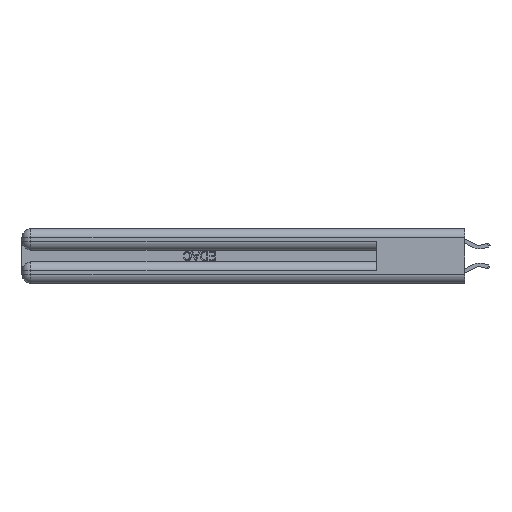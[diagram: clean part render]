
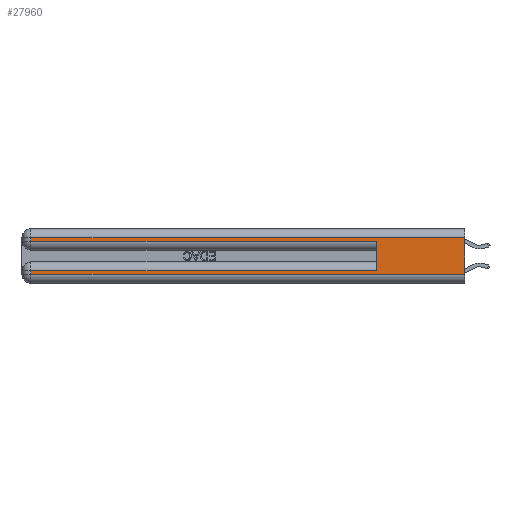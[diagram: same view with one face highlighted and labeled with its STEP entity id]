
A CAD part, left-side view. The second image highlights one B-rep face of the part: STEP entity #27960.
In plain terms, the highlighted planar face has unit normal (-1, 0, 0).
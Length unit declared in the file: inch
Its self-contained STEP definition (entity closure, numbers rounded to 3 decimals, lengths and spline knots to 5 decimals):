
#130 = LINE ( 'NONE', #24938, #30496 ) ;
#816 = LINE ( 'NONE', #9879, #31984 ) ;
#1373 = VECTOR ( 'NONE', #23966, 39.37008 ) ;
#2949 = DIRECTION ( 'NONE',  ( 0., 0., 1. ) ) ;
#3245 = EDGE_CURVE ( 'NONE', #4053, #3680, #5400, .T. ) ;
#3680 = VERTEX_POINT ( 'NONE', #26156 ) ;
#3933 = EDGE_CURVE ( 'NONE', #4053, #18647, #4117, .T. ) ;
#4053 = VERTEX_POINT ( 'NONE', #16327 ) ;
#4099 = CARTESIAN_POINT ( 'NONE',  ( 0., 2.94, 0.31 ) ) ;
#4117 = LINE ( 'NONE', #5490, #31559 ) ;
#4301 = CARTESIAN_POINT ( 'NONE',  ( 0., 0., 0.06 ) ) ;
#5032 = ORIENTED_EDGE ( 'NONE', *, *, #28928, .T. ) ;
#5400 = LINE ( 'NONE', #34355, #10817 ) ;
#5490 = CARTESIAN_POINT ( 'NONE',  ( 0., 0.6, 0.145 ) ) ;
#5714 = VERTEX_POINT ( 'NONE', #21683 ) ;
#5904 = VERTEX_POINT ( 'NONE', #4301 ) ;
#6257 = DIRECTION ( 'NONE',  ( 0., 0., -1. ) ) ;
#7238 = LINE ( 'NONE', #32750, #31319 ) ;
#7413 = DIRECTION ( 'NONE',  ( 0., -1., 0. ) ) ;
#7583 = CARTESIAN_POINT ( 'NONE',  ( 0., 2.94, 0.285 ) ) ;
#7612 = PLANE ( 'NONE',  #24743 ) ;
#7894 = DIRECTION ( 'NONE',  ( 0., 1., 0. ) ) ;
#8064 = CARTESIAN_POINT ( 'NONE',  ( 0., 0., 0.37 ) ) ;
#8297 = EDGE_CURVE ( 'NONE', #5714, #5904, #19740, .T. ) ;
#8478 = LINE ( 'NONE', #10328, #1373 ) ;
#9458 = ORIENTED_EDGE ( 'NONE', *, *, #3933, .F. ) ;
#9879 = CARTESIAN_POINT ( 'NONE',  ( 0., 0., 0.06 ) ) ;
#10328 = CARTESIAN_POINT ( 'NONE',  ( 0., 0., 0.285 ) ) ;
#10817 = VECTOR ( 'NONE', #7894, 39.37008 ) ;
#12127 = ORIENTED_EDGE ( 'NONE', *, *, #17957, .T. ) ;
#12734 = CARTESIAN_POINT ( 'NONE',  ( 0., 0.6, 0.285 ) ) ;
#13057 = EDGE_LOOP ( 'NONE', ( #14202, #24179, #12127, #20337, #9458, #28862, #5032, #24254 ) ) ;
#14202 = ORIENTED_EDGE ( 'NONE', *, *, #8297, .F. ) ;
#14277 = VECTOR ( 'NONE', #15119, 39.37008 ) ;
#14525 = DIRECTION ( 'NONE',  ( 0., 1., 0. ) ) ;
#14893 = LINE ( 'NONE', #17825, #34388 ) ;
#15119 = DIRECTION ( 'NONE',  ( 0., 0., -1. ) ) ;
#15748 = DIRECTION ( 'NONE',  ( 1., 0., 0. ) ) ;
#16327 = CARTESIAN_POINT ( 'NONE',  ( 0., 0.6, 0.085 ) ) ;
#17825 = CARTESIAN_POINT ( 'NONE',  ( 0., 2.94, 0.37 ) ) ;
#17957 = EDGE_CURVE ( 'NONE', #34346, #30354, #14893, .T. ) ;
#18294 = CARTESIAN_POINT ( 'NONE',  ( 0., 0., 0.37 ) ) ;
#18647 = VERTEX_POINT ( 'NONE', #12734 ) ;
#18986 = FACE_OUTER_BOUND ( 'NONE', #13057, .T. ) ;
#19740 = LINE ( 'NONE', #18294, #14277 ) ;
#20337 = ORIENTED_EDGE ( 'NONE', *, *, #32397, .T. ) ;
#20404 = DIRECTION ( 'NONE',  ( 0., 0., -1. ) ) ;
#21683 = CARTESIAN_POINT ( 'NONE',  ( 0., 0., 0.31 ) ) ;
#23126 = EDGE_CURVE ( 'NONE', #26968, #5904, #816, .T. ) ;
#23966 = DIRECTION ( 'NONE',  ( 0., -1., 0. ) ) ;
#24179 = ORIENTED_EDGE ( 'NONE', *, *, #28907, .T. ) ;
#24254 = ORIENTED_EDGE ( 'NONE', *, *, #23126, .T. ) ;
#24743 = AXIS2_PLACEMENT_3D ( 'NONE', #8064, #15748, #29121 ) ;
#24938 = CARTESIAN_POINT ( 'NONE',  ( 0., 0., 0.31 ) ) ;
#26156 = CARTESIAN_POINT ( 'NONE',  ( 0., 2.94, 0.085 ) ) ;
#26968 = VERTEX_POINT ( 'NONE', #33090 ) ;
#27960 = ADVANCED_FACE ( 'NONE', ( #18986 ), #7612, .F. ) ;
#28862 = ORIENTED_EDGE ( 'NONE', *, *, #3245, .T. ) ;
#28907 = EDGE_CURVE ( 'NONE', #5714, #34346, #130, .T. ) ;
#28928 = EDGE_CURVE ( 'NONE', #3680, #26968, #7238, .T. ) ;
#29121 = DIRECTION ( 'NONE',  ( 0., 0., -1. ) ) ;
#30354 = VERTEX_POINT ( 'NONE', #7583 ) ;
#30496 = VECTOR ( 'NONE', #14525, 39.37008 ) ;
#31319 = VECTOR ( 'NONE', #6257, 39.37008 ) ;
#31559 = VECTOR ( 'NONE', #2949, 39.37008 ) ;
#31984 = VECTOR ( 'NONE', #7413, 39.37008 ) ;
#32397 = EDGE_CURVE ( 'NONE', #30354, #18647, #8478, .T. ) ;
#32750 = CARTESIAN_POINT ( 'NONE',  ( 0., 2.94, 0.37 ) ) ;
#33090 = CARTESIAN_POINT ( 'NONE',  ( 0., 2.94, 0.06 ) ) ;
#34346 = VERTEX_POINT ( 'NONE', #4099 ) ;
#34355 = CARTESIAN_POINT ( 'NONE',  ( 0., 0., 0.085 ) ) ;
#34388 = VECTOR ( 'NONE', #20404, 39.37008 ) ;
